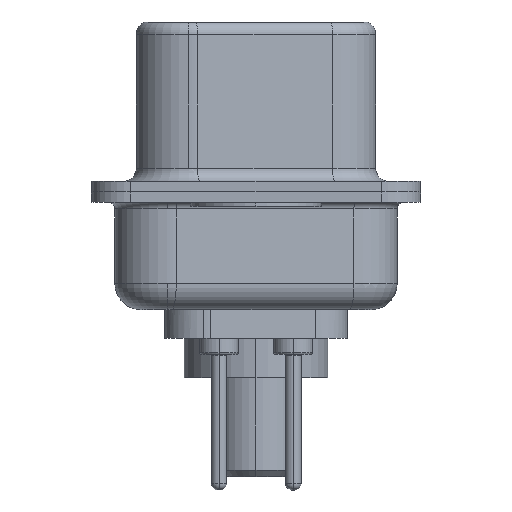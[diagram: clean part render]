
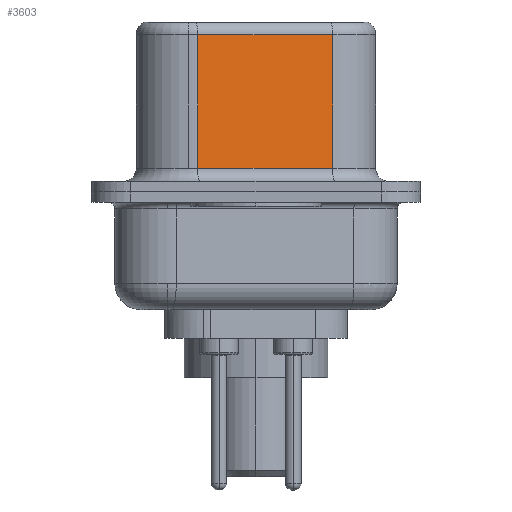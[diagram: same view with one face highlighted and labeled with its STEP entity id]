
A CAD part, left-side view. The second image highlights one B-rep face of the part: STEP entity #3603.
In plain terms, the highlighted planar face has unit normal (-0.985, -0.174, 0).
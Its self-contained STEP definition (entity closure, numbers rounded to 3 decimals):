
#77 = EDGE_CURVE ( 'NONE', #1544, #8109, #3278, .T. ) ;
#127 = CARTESIAN_POINT ( 'NONE',  ( 4.565, -2.927, 6.52 ) ) ;
#557 = CARTESIAN_POINT ( 'NONE',  ( 3.655, 2.233, 0.9 ) ) ;
#1542 = DIRECTION ( 'NONE',  ( 0.174, -0.985, 0. ) ) ;
#1544 = VERTEX_POINT ( 'NONE', #4125 ) ;
#1577 = LINE ( 'NONE', #2795, #12082 ) ;
#2188 = VECTOR ( 'NONE', #1542, 1000. ) ;
#2306 = DIRECTION ( 'NONE',  ( 0.985, 0.174, 0. ) ) ;
#2446 = PLANE ( 'NONE',  #14894 ) ;
#2748 = DIRECTION ( 'NONE',  ( 0., 0., -1. ) ) ;
#2795 = CARTESIAN_POINT ( 'NONE',  ( 3.655, 2.233, 6.52 ) ) ;
#3278 = LINE ( 'NONE', #9197, #9145 ) ;
#3290 = CARTESIAN_POINT ( 'NONE',  ( 3.655, 2.233, 6.02 ) ) ;
#3603 = ADVANCED_FACE ( 'NONE', ( #14236 ), #2446, .F. ) ;
#3931 = ORIENTED_EDGE ( 'NONE', *, *, #77, .T. ) ;
#4125 = CARTESIAN_POINT ( 'NONE',  ( 4.565, -2.927, 6.02 ) ) ;
#5891 = DIRECTION ( 'NONE',  ( -0.174, 0.985, 0. ) ) ;
#6292 = DIRECTION ( 'NONE',  ( 0., 0., -1. ) ) ;
#6604 = VERTEX_POINT ( 'NONE', #11427 ) ;
#7016 = ORIENTED_EDGE ( 'NONE', *, *, #7224, .F. ) ;
#7224 = EDGE_CURVE ( 'NONE', #1544, #6604, #12527, .T. ) ;
#7347 = CARTESIAN_POINT ( 'NONE',  ( 4.565, -2.927, 0.9 ) ) ;
#7462 = EDGE_LOOP ( 'NONE', ( #7016, #3931, #11276, #9431 ) ) ;
#8109 = VERTEX_POINT ( 'NONE', #3290 ) ;
#8292 = EDGE_CURVE ( 'NONE', #9377, #6604, #8759, .T. ) ;
#8759 = LINE ( 'NONE', #7347, #2188 ) ;
#9145 = VECTOR ( 'NONE', #15163, 1000. ) ;
#9197 = CARTESIAN_POINT ( 'NONE',  ( 4.565, -2.927, 6.02 ) ) ;
#9377 = VERTEX_POINT ( 'NONE', #557 ) ;
#9431 = ORIENTED_EDGE ( 'NONE', *, *, #8292, .T. ) ;
#10534 = EDGE_CURVE ( 'NONE', #8109, #9377, #1577, .T. ) ;
#11276 = ORIENTED_EDGE ( 'NONE', *, *, #10534, .T. ) ;
#11427 = CARTESIAN_POINT ( 'NONE',  ( 4.565, -2.927, 0.9 ) ) ;
#12082 = VECTOR ( 'NONE', #2748, 1000. ) ;
#12519 = CARTESIAN_POINT ( 'NONE',  ( 4.565, -2.927, 6.52 ) ) ;
#12527 = LINE ( 'NONE', #12519, #14900 ) ;
#14236 = FACE_OUTER_BOUND ( 'NONE', #7462, .T. ) ;
#14894 = AXIS2_PLACEMENT_3D ( 'NONE', #127, #2306, #5891 ) ;
#14900 = VECTOR ( 'NONE', #6292, 1000. ) ;
#15163 = DIRECTION ( 'NONE',  ( -0.174, 0.985, 0. ) ) ;
